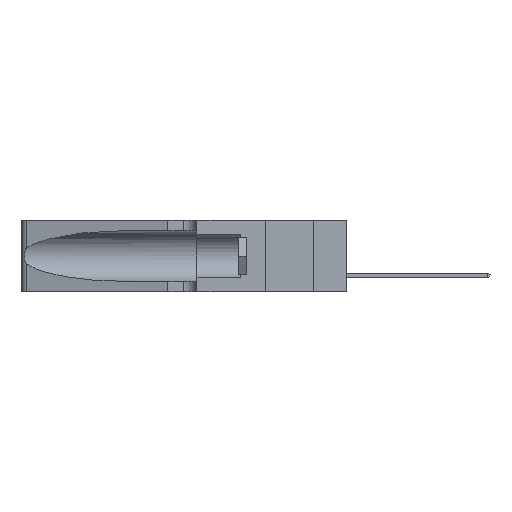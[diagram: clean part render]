
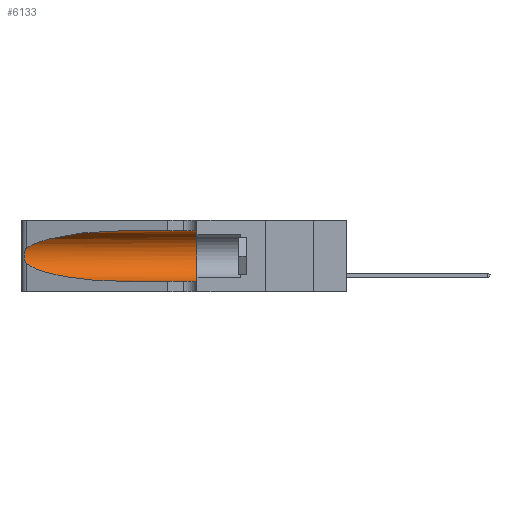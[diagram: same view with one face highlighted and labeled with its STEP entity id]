
A CAD part, left-side view. The second image highlights one B-rep face of the part: STEP entity #6133.
In plain terms, the highlighted cylindrical face has radius 3.308 mm (diameter 6.617 mm), a partial arc.
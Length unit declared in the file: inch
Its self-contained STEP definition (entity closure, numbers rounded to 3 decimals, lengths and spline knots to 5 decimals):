
#166 = CARTESIAN_POINT ( 'NONE',  ( 0.1305, 1.61858, 0.185 ) ) ;
#351 = CARTESIAN_POINT ( 'NONE',  ( 0.25487, 1.22718, 0.14631 ) ) ;
#859 = EDGE_LOOP ( 'NONE', ( #4669, #22943, #15751, #1210, #23785, #23650 ) ) ;
#1110 = VERTEX_POINT ( 'NONE', #5821 ) ;
#1210 = ORIENTED_EDGE ( 'NONE', *, *, #12077, .T. ) ;
#1232 = CIRCLE ( 'NONE', #24484, 0.13025 ) ;
#2149 = CARTESIAN_POINT ( 'NONE',  ( 0.1305, 0.72297, 0.31525 ) ) ;
#2593 = CARTESIAN_POINT ( 'NONE',  ( 0.26017, 1.23833, 0.17102 ) ) ;
#3972 = CARTESIAN_POINT ( 'NONE',  ( 0.18966, 0.96281, 0.31525 ) ) ;
#4669 = ORIENTED_EDGE ( 'NONE', *, *, #8570, .T. ) ;
#5300 = CARTESIAN_POINT ( 'NONE',  ( 0.1305, 0.72297, 0.31525 ) ) ;
#5821 = CARTESIAN_POINT ( 'NONE',  ( 0.1305, 0.35, 0.05475 ) ) ;
#6133 = ADVANCED_FACE ( 'NONE', ( #6704 ), #10131, .F. ) ;
#6140 = CARTESIAN_POINT ( 'NONE',  ( 0.1305, 0.35, 0.185 ) ) ;
#6225 = DIRECTION ( 'NONE',  ( 0., 0., 1. ) ) ;
#6462 = CARTESIAN_POINT ( 'NONE',  ( 0.25555, 1.22993, 0.14849 ) ) ;
#6562 = EDGE_CURVE ( 'NONE', #9240, #10876, #17815, .T. ) ;
#6627 = VERTEX_POINT ( 'NONE', #351 ) ;
#6704 = FACE_OUTER_BOUND ( 'NONE', #859, .T. ) ;
#6800 = DIRECTION ( 'NONE',  ( 0., -1., 0. ) ) ;
#8125 = CARTESIAN_POINT ( 'NONE',  ( 0.2373, 1.15595, 0.08982 ) ) ;
#8233 = B_SPLINE_CURVE_WITH_KNOTS ( 'NONE', 3,
 ( #18183, #18371, #10507, #10419, #12470, #14439, #8299, #22213, #2593, #16430, #12281, #14264, #6462, #16245 ),
 .UNSPECIFIED., .F., .F.,
 ( 4, 2, 2, 2, 2, 2, 4 ),
 ( 0., 0.00027, 0.00053, 0.00107, 0.0016, 0.00187, 0.00214 ),
 .UNSPECIFIED. ) ;
#8299 = CARTESIAN_POINT ( 'NONE',  ( 0.26075, 1.23896, 0.19203 ) ) ;
#8570 = EDGE_CURVE ( 'NONE', #9240, #25102, #19743, .T. ) ;
#9200 = EDGE_CURVE ( 'NONE', #6627, #17735, #12372, .T. ) ;
#9240 = VERTEX_POINT ( 'NONE', #2149 ) ;
#10131 = CYLINDRICAL_SURFACE ( 'NONE', #23606, 0.13025 ) ;
#10293 = DIRECTION ( 'NONE',  ( 0., 0., -1. ) ) ;
#10419 = CARTESIAN_POINT ( 'NONE',  ( 0.25787, 1.23484, 0.2124 ) ) ;
#10507 = CARTESIAN_POINT ( 'NONE',  ( 0.25639, 1.23184, 0.21858 ) ) ;
#10876 = VERTEX_POINT ( 'NONE', #19623 ) ;
#10995 = VECTOR ( 'NONE', #6800, 39.37008 ) ;
#11787 = CARTESIAN_POINT ( 'NONE',  ( 0.1305, 1.61858, 0.31525 ) ) ;
#12077 = EDGE_CURVE ( 'NONE', #17735, #1110, #25267, .T. ) ;
#12281 = CARTESIAN_POINT ( 'NONE',  ( 0.25789, 1.23486, 0.15765 ) ) ;
#12372 =( BOUNDED_CURVE ( )  B_SPLINE_CURVE ( 3, ( #19979, #8125, #13937, #22044 ),
 .UNSPECIFIED., .F., .T. ) 
 B_SPLINE_CURVE_WITH_KNOTS ( ( 4, 4 ),
 ( 3.44316, 4.71239 ),
 .UNSPECIFIED. ) 
 CURVE ( )  GEOMETRIC_REPRESENTATION_ITEM ( )  RATIONAL_B_SPLINE_CURVE ( ( 1., 0.87, 0.87, 1. ) ) 
 REPRESENTATION_ITEM ( '' )  );
#12470 = CARTESIAN_POINT ( 'NONE',  ( 0.25854, 1.2359, 0.20912 ) ) ;
#13785 = VECTOR ( 'NONE', #14015, 39.37008 ) ;
#13841 = CARTESIAN_POINT ( 'NONE',  ( 0.2373, 1.15595, 0.28018 ) ) ;
#13937 = CARTESIAN_POINT ( 'NONE',  ( 0.18966, 0.96281, 0.05475 ) ) ;
#14015 = DIRECTION ( 'NONE',  ( 0., -1., 0. ) ) ;
#14264 = CARTESIAN_POINT ( 'NONE',  ( 0.25639, 1.23186, 0.15144 ) ) ;
#14439 = CARTESIAN_POINT ( 'NONE',  ( 0.26018, 1.23835, 0.19895 ) ) ;
#14742 = CARTESIAN_POINT ( 'NONE',  ( 0.1305, 1.61858, 0.05475 ) ) ;
#15751 = ORIENTED_EDGE ( 'NONE', *, *, #9200, .T. ) ;
#15959 = CARTESIAN_POINT ( 'NONE',  ( 0.25487, 1.22718, 0.22369 ) ) ;
#16245 = CARTESIAN_POINT ( 'NONE',  ( 0.25487, 1.22718, 0.14631 ) ) ;
#16430 = CARTESIAN_POINT ( 'NONE',  ( 0.25856, 1.23593, 0.16098 ) ) ;
#17735 = VERTEX_POINT ( 'NONE', #24891 ) ;
#17815 = LINE ( 'NONE', #11787, #13785 ) ;
#17835 = CARTESIAN_POINT ( 'NONE',  ( 0.25487, 1.22718, 0.22369 ) ) ;
#18005 = EDGE_CURVE ( 'NONE', #10876, #1110, #1232, .T. ) ;
#18183 = CARTESIAN_POINT ( 'NONE',  ( 0.25487, 1.22718, 0.22369 ) ) ;
#18371 = CARTESIAN_POINT ( 'NONE',  ( 0.25555, 1.22994, 0.2215 ) ) ;
#19623 = CARTESIAN_POINT ( 'NONE',  ( 0.1305, 0.35, 0.31525 ) ) ;
#19678 = EDGE_CURVE ( 'NONE', #25102, #6627, #8233, .T. ) ;
#19743 =( BOUNDED_CURVE ( )  B_SPLINE_CURVE ( 3, ( #5300, #3972, #13841, #17835 ),
 .UNSPECIFIED., .F., .F. ) 
 B_SPLINE_CURVE_WITH_KNOTS ( ( 4, 4 ),
 ( 1.5708, 2.84003 ),
 .UNSPECIFIED. ) 
 CURVE ( )  GEOMETRIC_REPRESENTATION_ITEM ( )  RATIONAL_B_SPLINE_CURVE ( ( 1., 0.87, 0.87, 1. ) ) 
 REPRESENTATION_ITEM ( '' )  );
#19979 = CARTESIAN_POINT ( 'NONE',  ( 0.25487, 1.22718, 0.14631 ) ) ;
#22044 = CARTESIAN_POINT ( 'NONE',  ( 0.1305, 0.72297, 0.05475 ) ) ;
#22066 = DIRECTION ( 'NONE',  ( 0., 1., 0. ) ) ;
#22173 = DIRECTION ( 'NONE',  ( 0., -1., 0. ) ) ;
#22213 = CARTESIAN_POINT ( 'NONE',  ( 0.26075, 1.23896, 0.178 ) ) ;
#22943 = ORIENTED_EDGE ( 'NONE', *, *, #19678, .T. ) ;
#23606 = AXIS2_PLACEMENT_3D ( 'NONE', #166, #22173, #10293 ) ;
#23650 = ORIENTED_EDGE ( 'NONE', *, *, #6562, .F. ) ;
#23785 = ORIENTED_EDGE ( 'NONE', *, *, #18005, .F. ) ;
#24484 = AXIS2_PLACEMENT_3D ( 'NONE', #6140, #22066, #6225 ) ;
#24891 = CARTESIAN_POINT ( 'NONE',  ( 0.1305, 0.72297, 0.05475 ) ) ;
#25102 = VERTEX_POINT ( 'NONE', #15959 ) ;
#25267 = LINE ( 'NONE', #14742, #10995 ) ;
